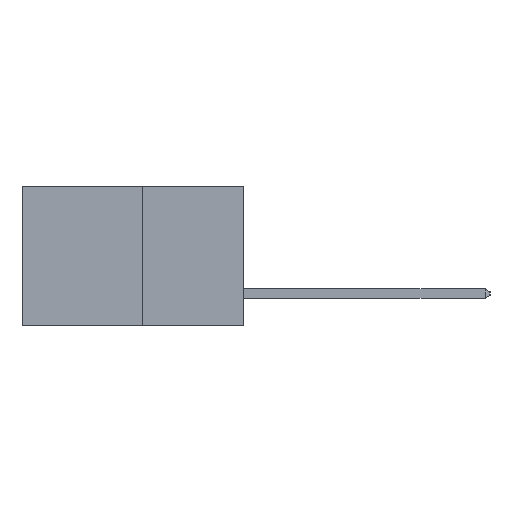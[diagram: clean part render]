
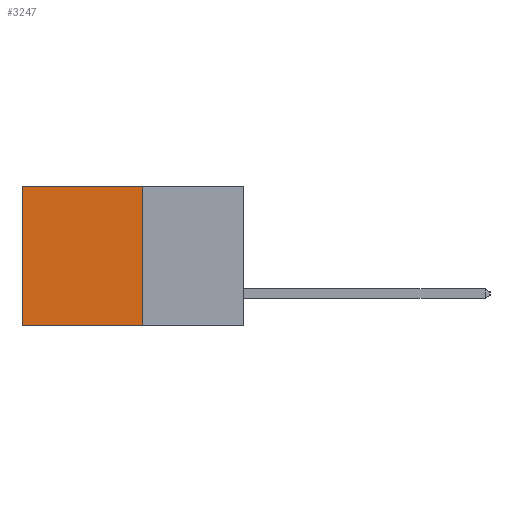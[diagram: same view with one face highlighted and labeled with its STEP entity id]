
A CAD part, left-side view. The second image highlights one B-rep face of the part: STEP entity #3247.
In plain terms, the highlighted planar face has unit normal (-1, 0, 0).
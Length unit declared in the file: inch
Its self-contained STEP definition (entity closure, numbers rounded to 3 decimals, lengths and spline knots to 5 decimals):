
#1557 = CARTESIAN_POINT ( 'NONE',  ( 0.277, 0.27, -0.37 ) ) ;
#1623 = CARTESIAN_POINT ( 'NONE',  ( 0.277, 0.59, -0.37 ) ) ;
#1638 = AXIS2_PLACEMENT_3D ( 'NONE', #1557, #15230, #15210 ) ;
#2185 = VERTEX_POINT ( 'NONE', #8522 ) ;
#2561 = ORIENTED_EDGE ( 'NONE', *, *, #15546, .F. ) ;
#3247 = ADVANCED_FACE ( 'NONE', ( #18606 ), #19775, .F. ) ;
#3286 = VERTEX_POINT ( 'NONE', #16235 ) ;
#6703 = CARTESIAN_POINT ( 'NONE',  ( 0.277, 0.27, -0.37 ) ) ;
#7249 = EDGE_CURVE ( 'NONE', #3286, #2185, #7619, .T. ) ;
#7619 = LINE ( 'NONE', #7823, #21053 ) ;
#7823 = CARTESIAN_POINT ( 'NONE',  ( 0.277, 0.27, 0. ) ) ;
#8106 = ORIENTED_EDGE ( 'NONE', *, *, #14308, .F. ) ;
#8196 = DIRECTION ( 'NONE',  ( 0., 1., 0. ) ) ;
#8522 = CARTESIAN_POINT ( 'NONE',  ( 0.277, 0.59, 0. ) ) ;
#9762 = CARTESIAN_POINT ( 'NONE',  ( 0.277, 0.27, -0.37 ) ) ;
#10144 = LINE ( 'NONE', #13397, #13582 ) ;
#10263 = VERTEX_POINT ( 'NONE', #1623 ) ;
#10498 = VECTOR ( 'NONE', #11972, 39.37008 ) ;
#11597 = LINE ( 'NONE', #6703, #16585 ) ;
#11667 = DIRECTION ( 'NONE',  ( 0., 0., -1. ) ) ;
#11972 = DIRECTION ( 'NONE',  ( 0., 0., -1. ) ) ;
#12235 = ORIENTED_EDGE ( 'NONE', *, *, #7249, .T. ) ;
#12947 = VERTEX_POINT ( 'NONE', #9762 ) ;
#13397 = CARTESIAN_POINT ( 'NONE',  ( 0.277, 0.59, -0.37 ) ) ;
#13582 = VECTOR ( 'NONE', #11667, 39.37008 ) ;
#14308 = EDGE_CURVE ( 'NONE', #12947, #10263, #11597, .T. ) ;
#14956 = LINE ( 'NONE', #15208, #10498 ) ;
#15208 = CARTESIAN_POINT ( 'NONE',  ( 0.277, 0.27, -0.37 ) ) ;
#15210 = DIRECTION ( 'NONE',  ( 0., 0., -1. ) ) ;
#15230 = DIRECTION ( 'NONE',  ( 1., 0., 0. ) ) ;
#15546 = EDGE_CURVE ( 'NONE', #3286, #12947, #14956, .T. ) ;
#16235 = CARTESIAN_POINT ( 'NONE',  ( 0.277, 0.27, 0. ) ) ;
#16585 = VECTOR ( 'NONE', #21824, 39.37008 ) ;
#17007 = EDGE_LOOP ( 'NONE', ( #20739, #8106, #2561, #12235 ) ) ;
#17492 = EDGE_CURVE ( 'NONE', #2185, #10263, #10144, .T. ) ;
#18606 = FACE_OUTER_BOUND ( 'NONE', #17007, .T. ) ;
#19775 = PLANE ( 'NONE',  #1638 ) ;
#20739 = ORIENTED_EDGE ( 'NONE', *, *, #17492, .T. ) ;
#21053 = VECTOR ( 'NONE', #8196, 39.37008 ) ;
#21824 = DIRECTION ( 'NONE',  ( 0., 1., 0. ) ) ;
